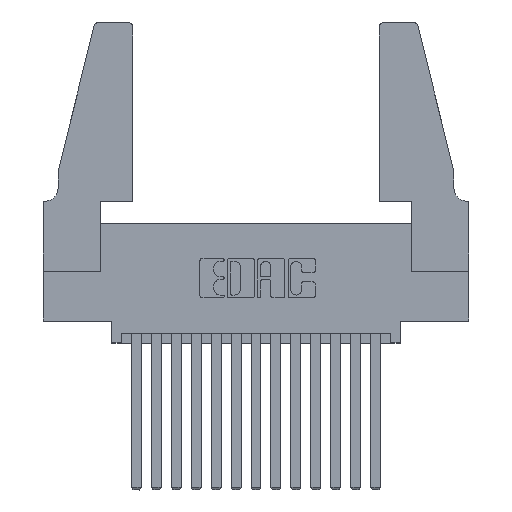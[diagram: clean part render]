
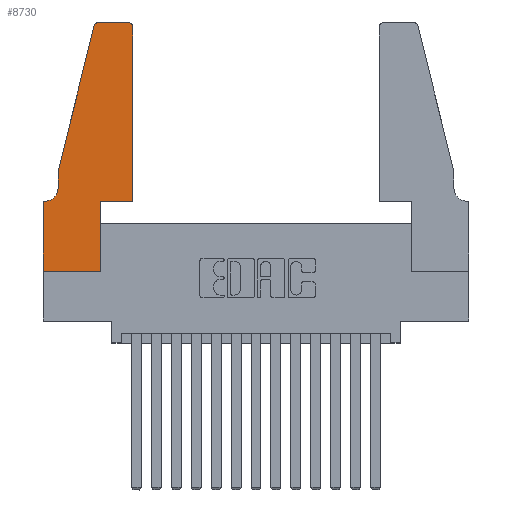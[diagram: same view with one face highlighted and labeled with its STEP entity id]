
A CAD part, top view. The second image highlights one B-rep face of the part: STEP entity #8730.
In plain terms, the highlighted planar face has unit normal (0, 0, 1).
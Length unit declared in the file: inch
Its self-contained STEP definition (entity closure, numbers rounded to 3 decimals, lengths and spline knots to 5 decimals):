
#263 = EDGE_CURVE ( 'NONE', #3178, #15811, #2498, .T. ) ;
#458 = VECTOR ( 'NONE', #5961, 39.37008 ) ;
#562 = DIRECTION ( 'NONE',  ( 1., 0., 0. ) ) ;
#643 = VERTEX_POINT ( 'NONE', #5629 ) ;
#1180 = DIRECTION ( 'NONE',  ( 1., 0., 0. ) ) ;
#1262 = CARTESIAN_POINT ( 'NONE',  ( 0., 0., 0.37 ) ) ;
#1430 = LINE ( 'NONE', #1523, #9081 ) ;
#1480 = CARTESIAN_POINT ( 'NONE',  ( 0.4505, 1.22, 0.37 ) ) ;
#1523 = CARTESIAN_POINT ( 'NONE',  ( 0.4505, 0.35, 0.37 ) ) ;
#1640 = VECTOR ( 'NONE', #8102, 39.37008 ) ;
#1642 = ORIENTED_EDGE ( 'NONE', *, *, #8034, .T. ) ;
#1843 = VECTOR ( 'NONE', #1180, 39.37008 ) ;
#2071 = EDGE_CURVE ( 'NONE', #14415, #7778, #3783, .T. ) ;
#2160 = LINE ( 'NONE', #10510, #6275 ) ;
#2397 = FACE_OUTER_BOUND ( 'NONE', #4847, .T. ) ;
#2455 = EDGE_CURVE ( 'NONE', #6227, #16219, #8896, .T. ) ;
#2498 = CIRCLE ( 'NONE', #7292, 0.03 ) ;
#2703 = DIRECTION ( 'NONE',  ( 0., 0., 1. ) ) ;
#2710 = EDGE_CURVE ( 'NONE', #15081, #14415, #6715, .T. ) ;
#2979 = DIRECTION ( 'NONE',  ( -0.239, -0.971, 0. ) ) ;
#2991 = ORIENTED_EDGE ( 'NONE', *, *, #263, .T. ) ;
#3151 = CARTESIAN_POINT ( 'NONE',  ( 0.0755, 0.5, 0.37 ) ) ;
#3178 = VERTEX_POINT ( 'NONE', #1480 ) ;
#3179 = EDGE_CURVE ( 'NONE', #7778, #14566, #14916, .T. ) ;
#3374 = VECTOR ( 'NONE', #8729, 39.37008 ) ;
#3486 = CARTESIAN_POINT ( 'NONE',  ( 0.4505, 0.35, 0.37 ) ) ;
#3595 = LINE ( 'NONE', #9688, #10468 ) ;
#3669 = CARTESIAN_POINT ( 'NONE',  ( 0.0755, 0.5, 0.37 ) ) ;
#3783 = LINE ( 'NONE', #12471, #1843 ) ;
#3846 = CARTESIAN_POINT ( 'NONE',  ( 0.4205, 1.22, 0.37 ) ) ;
#4036 = CARTESIAN_POINT ( 'NONE',  ( 0.2865, 0.35, 0.37 ) ) ;
#4290 = AXIS2_PLACEMENT_3D ( 'NONE', #9115, #9172, #12779 ) ;
#4465 = ORIENTED_EDGE ( 'NONE', *, *, #6436, .T. ) ;
#4498 = VECTOR ( 'NONE', #2979, 39.37008 ) ;
#4545 = CARTESIAN_POINT ( 'NONE',  ( 0.284, 1.25, 0.37 ) ) ;
#4669 = DIRECTION ( 'NONE',  ( -1., 0., 0. ) ) ;
#4753 = EDGE_CURVE ( 'NONE', #7834, #6227, #9029, .T. ) ;
#4847 = EDGE_LOOP ( 'NONE', ( #12624, #4465, #8288, #14126, #14798, #15122, #8796, #14447, #9190, #5243, #1642, #2991 ) ) ;
#5243 = ORIENTED_EDGE ( 'NONE', *, *, #12913, .T. ) ;
#5629 = CARTESIAN_POINT ( 'NONE',  ( 0.4505, 0.35, 0.37 ) ) ;
#5662 = DIRECTION ( 'NONE',  ( 0., 1., 0. ) ) ;
#5961 = DIRECTION ( 'NONE',  ( 1., 0., 0. ) ) ;
#5962 = CARTESIAN_POINT ( 'NONE',  ( 0.2865, 0., 0.37 ) ) ;
#6022 = CARTESIAN_POINT ( 'NONE',  ( 0.0055, 0.35, 0.37 ) ) ;
#6123 = CARTESIAN_POINT ( 'NONE',  ( 0.25487, 1.22718, 0.37 ) ) ;
#6227 = VERTEX_POINT ( 'NONE', #3669 ) ;
#6275 = VECTOR ( 'NONE', #13155, 39.37008 ) ;
#6436 = EDGE_CURVE ( 'NONE', #10865, #7834, #7691, .T. ) ;
#6478 = EDGE_CURVE ( 'NONE', #16219, #6953, #12865, .T. ) ;
#6715 = LINE ( 'NONE', #1262, #3374 ) ;
#6953 = VERTEX_POINT ( 'NONE', #6022 ) ;
#7292 = AXIS2_PLACEMENT_3D ( 'NONE', #3846, #12524, #10118 ) ;
#7367 = AXIS2_PLACEMENT_3D ( 'NONE', #10154, #2703, #15027 ) ;
#7525 = EDGE_CURVE ( 'NONE', #6953, #15081, #3595, .T. ) ;
#7691 = CIRCLE ( 'NONE', #7367, 0.03 ) ;
#7778 = VERTEX_POINT ( 'NONE', #5962 ) ;
#7834 = VERTEX_POINT ( 'NONE', #6123 ) ;
#7989 = CARTESIAN_POINT ( 'NONE',  ( 0.0755, 0.5, 0.37 ) ) ;
#8034 = EDGE_CURVE ( 'NONE', #643, #3178, #1430, .T. ) ;
#8102 = DIRECTION ( 'NONE',  ( 0., -1., 0. ) ) ;
#8288 = ORIENTED_EDGE ( 'NONE', *, *, #4753, .T. ) ;
#8508 = CARTESIAN_POINT ( 'NONE',  ( 0.4205, 1.25, 0.37 ) ) ;
#8729 = DIRECTION ( 'NONE',  ( 0., -1., 0. ) ) ;
#8730 = ADVANCED_FACE ( 'NONE', ( #2397 ), #15573, .T. ) ;
#8796 = ORIENTED_EDGE ( 'NONE', *, *, #2710, .T. ) ;
#8896 = LINE ( 'NONE', #3151, #1640 ) ;
#9029 = LINE ( 'NONE', #7989, #4498 ) ;
#9030 = CARTESIAN_POINT ( 'NONE',  ( 0., 0., 0.37 ) ) ;
#9081 = VECTOR ( 'NONE', #5662, 39.37008 ) ;
#9115 = CARTESIAN_POINT ( 'NONE',  ( 0.0055, 0.42, 0.37 ) ) ;
#9172 = DIRECTION ( 'NONE',  ( 0., 0., -1. ) ) ;
#9190 = ORIENTED_EDGE ( 'NONE', *, *, #3179, .T. ) ;
#9688 = CARTESIAN_POINT ( 'NONE',  ( 0.0755, 0.35, 0.37 ) ) ;
#10032 = EDGE_CURVE ( 'NONE', #15811, #10865, #2160, .T. ) ;
#10118 = DIRECTION ( 'NONE',  ( 1., 0., 0. ) ) ;
#10154 = CARTESIAN_POINT ( 'NONE',  ( 0.284, 1.22, 0.37 ) ) ;
#10468 = VECTOR ( 'NONE', #4669, 39.37008 ) ;
#10510 = CARTESIAN_POINT ( 'NONE',  ( 0.2605, 1.25, 0.37 ) ) ;
#10580 = DIRECTION ( 'NONE',  ( 0., 0., 1. ) ) ;
#10865 = VERTEX_POINT ( 'NONE', #4545 ) ;
#11123 = AXIS2_PLACEMENT_3D ( 'NONE', #14423, #10580, #562 ) ;
#12031 = LINE ( 'NONE', #3486, #458 ) ;
#12173 = CARTESIAN_POINT ( 'NONE',  ( 0., 0.35, 0.37 ) ) ;
#12471 = CARTESIAN_POINT ( 'NONE',  ( 0., 0., 0.37 ) ) ;
#12524 = DIRECTION ( 'NONE',  ( 0., 0., 1. ) ) ;
#12624 = ORIENTED_EDGE ( 'NONE', *, *, #10032, .T. ) ;
#12779 = DIRECTION ( 'NONE',  ( -1., 0., 0. ) ) ;
#12865 = CIRCLE ( 'NONE', #4290, 0.07 ) ;
#12913 = EDGE_CURVE ( 'NONE', #14566, #643, #12031, .T. ) ;
#12972 = VECTOR ( 'NONE', #15406, 39.37008 ) ;
#13155 = DIRECTION ( 'NONE',  ( -1., 0., 0. ) ) ;
#14126 = ORIENTED_EDGE ( 'NONE', *, *, #2455, .T. ) ;
#14351 = CARTESIAN_POINT ( 'NONE',  ( 0.2865, 0.35, 0.37 ) ) ;
#14415 = VERTEX_POINT ( 'NONE', #9030 ) ;
#14423 = CARTESIAN_POINT ( 'NONE',  ( 0., 0.35, 0.37 ) ) ;
#14447 = ORIENTED_EDGE ( 'NONE', *, *, #2071, .T. ) ;
#14566 = VERTEX_POINT ( 'NONE', #14351 ) ;
#14798 = ORIENTED_EDGE ( 'NONE', *, *, #6478, .T. ) ;
#14916 = LINE ( 'NONE', #4036, #12972 ) ;
#15027 = DIRECTION ( 'NONE',  ( 1., 0., 0. ) ) ;
#15081 = VERTEX_POINT ( 'NONE', #12173 ) ;
#15122 = ORIENTED_EDGE ( 'NONE', *, *, #7525, .T. ) ;
#15397 = CARTESIAN_POINT ( 'NONE',  ( 0.0755, 0.42, 0.37 ) ) ;
#15406 = DIRECTION ( 'NONE',  ( 0., 1., 0. ) ) ;
#15573 = PLANE ( 'NONE',  #11123 ) ;
#15811 = VERTEX_POINT ( 'NONE', #8508 ) ;
#16219 = VERTEX_POINT ( 'NONE', #15397 ) ;
